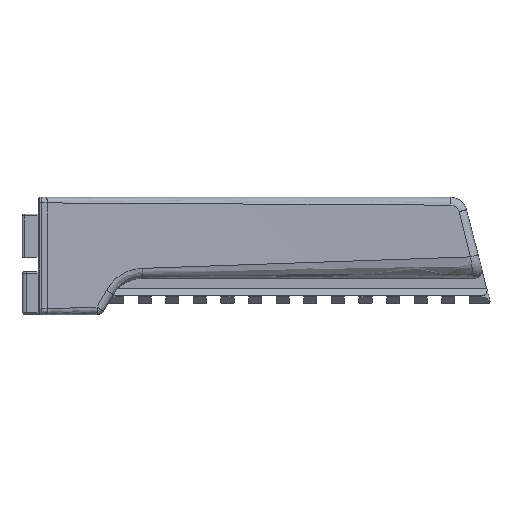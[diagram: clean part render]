
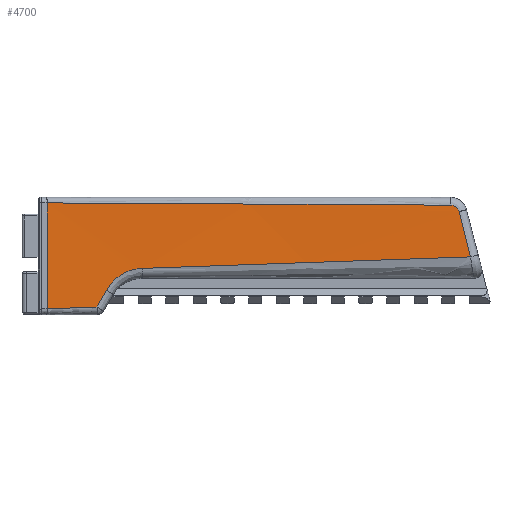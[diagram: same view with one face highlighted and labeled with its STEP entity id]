
A CAD part, left-side view. The second image highlights one B-rep face of the part: STEP entity #4700.
In plain terms, the highlighted cylindrical face has radius 3919.49 mm (diameter 7838.97 mm), a partial arc.
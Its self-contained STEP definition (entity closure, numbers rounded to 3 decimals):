
#278=CYLINDRICAL_SURFACE('',#5062,3919.486);
#595=LINE('',#9063,#1027);
#1027=VECTOR('',#5934,10.);
#1308=FACE_OUTER_BOUND('',#1581,.T.);
#1581=EDGE_LOOP('',(#3850,#3851,#3852,#3853,#3854,#3855,#3856,#3857));
#1857=B_SPLINE_CURVE_WITH_KNOTS('',3,(#8658,#8659,#8660,#8661,#8662,#8663),
 .UNSPECIFIED.,.F.,.F.,(4,1,1,4),(0.315,6.59,11.819,
14.956),.UNSPECIFIED.);
#1859=B_SPLINE_CURVE_WITH_KNOTS('',3,(#8707,#8708,#8709,#8710,#8711),
 .UNSPECIFIED.,.F.,.F.,(4,1,4),(14.956,15.135,15.373),
 .UNSPECIFIED.);
#1861=B_SPLINE_CURVE_WITH_KNOTS('',3,(#8743,#8744,#8745,#8746),
 .UNSPECIFIED.,.F.,.F.,(4,4),(15.373,17.059),
 .UNSPECIFIED.);
#1867=B_SPLINE_CURVE_WITH_KNOTS('',3,(#9050,#9051,#9052,#9053),
 .UNSPECIFIED.,.F.,.F.,(4,4),(-14.238,-2.308),
 .UNSPECIFIED.);
#1869=B_SPLINE_CURVE_WITH_KNOTS('',3,(#9065,#9066,#9067,#9068),
 .UNSPECIFIED.,.F.,.F.,(4,4),(-2.131,-0.315),
 .UNSPECIFIED.);
#1870=B_SPLINE_CURVE_WITH_KNOTS('',3,(#9070,#9071,#9072,#9073),
 .UNSPECIFIED.,.F.,.F.,(4,4),(-0.716,-0.017),
 .UNSPECIFIED.);
#1871=B_SPLINE_CURVE_WITH_KNOTS('',3,(#9074,#9075,#9076,#9077,#9078),
 .UNSPECIFIED.,.F.,.F.,(4,1,4),(-2.308,-1.398,-0.716),
 .UNSPECIFIED.);
#2273=VERTEX_POINT('',#8596);
#2274=VERTEX_POINT('',#8650);
#2275=VERTEX_POINT('',#8699);
#2276=VERTEX_POINT('',#8736);
#2281=VERTEX_POINT('',#9049);
#2282=VERTEX_POINT('',#9062);
#2283=VERTEX_POINT('',#9064);
#2284=VERTEX_POINT('',#9069);
#2856=EDGE_CURVE('',#2273,#2274,#1857,.T.);
#2858=EDGE_CURVE('',#2274,#2275,#1859,.T.);
#2860=EDGE_CURVE('',#2275,#2276,#1861,.T.);
#2868=EDGE_CURVE('',#2276,#2281,#1867,.T.);
#2870=EDGE_CURVE('',#2282,#2273,#595,.T.);
#2871=EDGE_CURVE('',#2283,#2282,#1869,.T.);
#2872=EDGE_CURVE('',#2284,#2283,#1870,.T.);
#2873=EDGE_CURVE('',#2281,#2284,#1871,.T.);
#3850=ORIENTED_EDGE('',*,*,#2860,.F.);
#3851=ORIENTED_EDGE('',*,*,#2858,.F.);
#3852=ORIENTED_EDGE('',*,*,#2856,.F.);
#3853=ORIENTED_EDGE('',*,*,#2870,.F.);
#3854=ORIENTED_EDGE('',*,*,#2871,.F.);
#3855=ORIENTED_EDGE('',*,*,#2872,.F.);
#3856=ORIENTED_EDGE('',*,*,#2873,.F.);
#3857=ORIENTED_EDGE('',*,*,#2868,.F.);
#4700=ADVANCED_FACE('',(#1308),#278,.F.);
#5062=AXIS2_PLACEMENT_3D('',#9061,#5932,#5933);
#5932=DIRECTION('center_axis',(0.,0.,1.));
#5933=DIRECTION('ref_axis',(0.998,0.063,0.));
#5934=DIRECTION('',(0.,0.,1.));
#8596=CARTESIAN_POINT('',(-9.04,-29.276,-116.917));
#8650=CARTESIAN_POINT('',(-2.521,-175.437,-117.725));
#8658=CARTESIAN_POINT('Ctrl Pts',(-9.04,-29.276,-116.917));
#8659=CARTESIAN_POINT('Ctrl Pts',(-7.719,-50.137,-117.032));
#8660=CARTESIAN_POINT('Ctrl Pts',(-5.603,-88.401,-117.244));
#8661=CARTESIAN_POINT('Ctrl Pts',(-3.625,-137.14,-117.513));
#8662=CARTESIAN_POINT('Ctrl Pts',(-2.792,-164.984,-117.667));
#8663=CARTESIAN_POINT('Ctrl Pts',(-2.521,-175.437,-117.725));
#8699=CARTESIAN_POINT('',(-2.444,-178.486,-120.11));
#8707=CARTESIAN_POINT('Ctrl Pts',(-2.521,-175.437,-117.725));
#8708=CARTESIAN_POINT('Ctrl Pts',(-2.506,-176.032,-117.728));
#8709=CARTESIAN_POINT('Ctrl Pts',(-2.47,-177.419,-118.136));
#8710=CARTESIAN_POINT('Ctrl Pts',(-2.448,-178.292,-119.339));
#8711=CARTESIAN_POINT('Ctrl Pts',(-2.444,-178.486,-120.11));
#8736=CARTESIAN_POINT('',(-2.342,-182.62,-136.458));
#8743=CARTESIAN_POINT('Ctrl Pts',(-2.444,-178.486,-120.11));
#8744=CARTESIAN_POINT('Ctrl Pts',(-2.409,-179.866,-125.567));
#8745=CARTESIAN_POINT('Ctrl Pts',(-2.375,-181.242,-131.007));
#8746=CARTESIAN_POINT('Ctrl Pts',(-2.342,-182.62,-136.458));
#9049=CARTESIAN_POINT('',(-7.01,-63.736,-140.621));
#9050=CARTESIAN_POINT('Ctrl Pts',(-2.342,-182.62,-136.458));
#9051=CARTESIAN_POINT('Ctrl Pts',(-3.296,-142.989,-137.846));
#9052=CARTESIAN_POINT('Ctrl Pts',(-4.851,-103.377,-139.233));
#9053=CARTESIAN_POINT('Ctrl Pts',(-7.01,-63.736,-140.621));
#9061=CARTESIAN_POINT('Origin',(-3920.692,-276.959,-114.899));
#9062=CARTESIAN_POINT('',(-9.04,-29.276,-155.275));
#9063=CARTESIAN_POINT('',(-9.04,-29.276,-114.899));
#9064=CARTESIAN_POINT('',(-7.936,-47.368,-154.622));
#9065=CARTESIAN_POINT('Ctrl Pts',(-7.936,-47.368,-154.622));
#9066=CARTESIAN_POINT('Ctrl Pts',(-8.29,-41.336,-154.84));
#9067=CARTESIAN_POINT('Ctrl Pts',(-8.658,-35.306,-155.057));
#9068=CARTESIAN_POINT('Ctrl Pts',(-9.04,-29.276,-155.275));
#9069=CARTESIAN_POINT('',(-7.739,-50.754,-148.518));
#9070=CARTESIAN_POINT('Ctrl Pts',(-7.739,-50.754,-148.518));
#9071=CARTESIAN_POINT('Ctrl Pts',(-7.804,-49.625,-150.553));
#9072=CARTESIAN_POINT('Ctrl Pts',(-7.87,-48.497,-152.587));
#9073=CARTESIAN_POINT('Ctrl Pts',(-7.936,-47.368,-154.622));
#9074=CARTESIAN_POINT('Ctrl Pts',(-7.01,-63.736,-140.621));
#9075=CARTESIAN_POINT('Ctrl Pts',(-7.175,-60.713,-140.727));
#9076=CARTESIAN_POINT('Ctrl Pts',(-7.467,-55.485,-142.485));
#9077=CARTESIAN_POINT('Ctrl Pts',(-7.676,-51.856,-146.532));
#9078=CARTESIAN_POINT('Ctrl Pts',(-7.739,-50.754,-148.518));
